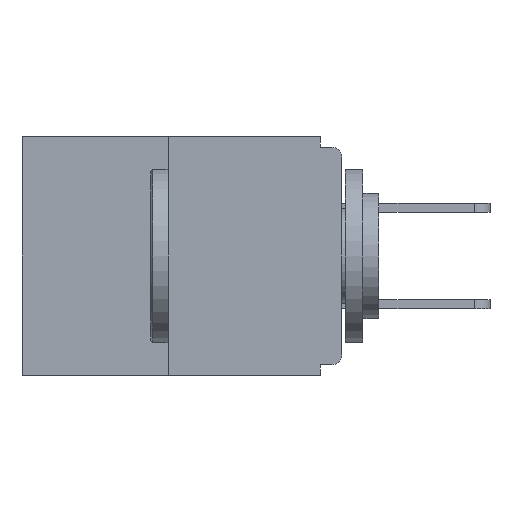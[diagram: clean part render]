
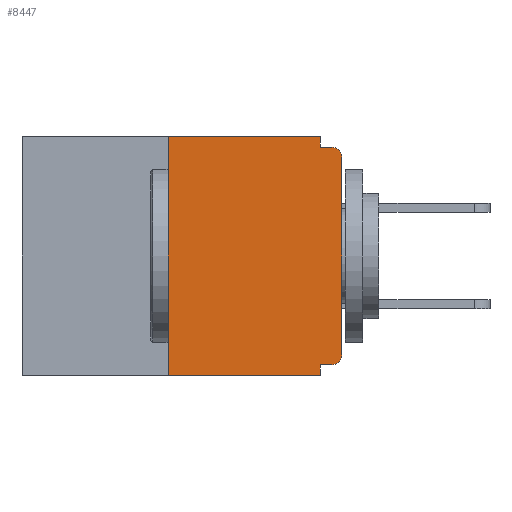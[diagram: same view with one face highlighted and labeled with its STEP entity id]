
A CAD part, left-side view. The second image highlights one B-rep face of the part: STEP entity #8447.
In plain terms, the highlighted planar face has unit normal (-1, 0, 0).
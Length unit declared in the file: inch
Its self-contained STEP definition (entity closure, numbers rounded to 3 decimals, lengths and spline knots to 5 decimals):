
#689 = LINE ( 'NONE', #3879, #4728 ) ;
#1601 = DIRECTION ( 'NONE',  ( 0., 0., -1. ) ) ;
#1775 = VECTOR ( 'NONE', #1817, 39.37008 ) ;
#1817 = DIRECTION ( 'NONE',  ( 0., 0., 1. ) ) ;
#2241 = LINE ( 'NONE', #26391, #17883 ) ;
#3178 = VECTOR ( 'NONE', #17143, 39.37008 ) ;
#3440 = CARTESIAN_POINT ( 'NONE',  ( 0., 0.25, 0. ) ) ;
#3879 = CARTESIAN_POINT ( 'NONE',  ( 0., 0.46, -0.343 ) ) ;
#4091 = LINE ( 'NONE', #7832, #24764 ) ;
#4187 = ORIENTED_EDGE ( 'NONE', *, *, #27512, .F. ) ;
#4209 = DIRECTION ( 'NONE',  ( 0., -1., 0. ) ) ;
#4233 = ORIENTED_EDGE ( 'NONE', *, *, #19570, .F. ) ;
#4329 = CIRCLE ( 'NONE', #6587, 0.015 ) ;
#4728 = VECTOR ( 'NONE', #22437, 39.37008 ) ;
#4934 = EDGE_CURVE ( 'NONE', #9540, #29131, #4329, .T. ) ;
#5716 = CIRCLE ( 'NONE', #19223, 0.015 ) ;
#5786 = EDGE_LOOP ( 'NONE', ( #4187, #16354, #23228, #4233, #12359, #24654, #11772, #14739, #16747, #27413 ) ) ;
#5897 = VERTEX_POINT ( 'NONE', #22244 ) ;
#6348 = CARTESIAN_POINT ( 'NONE',  ( 0., 0., -0.015 ) ) ;
#6507 = DIRECTION ( 'NONE',  ( -1., 0., 0. ) ) ;
#6508 = CARTESIAN_POINT ( 'NONE',  ( 0., 0.031, 0. ) ) ;
#6549 = CARTESIAN_POINT ( 'NONE',  ( 0., 0.015, -0.328 ) ) ;
#6587 = AXIS2_PLACEMENT_3D ( 'NONE', #12841, #15266, #22357 ) ;
#6956 = VERTEX_POINT ( 'NONE', #29626 ) ;
#7216 = VERTEX_POINT ( 'NONE', #6508 ) ;
#7235 = VECTOR ( 'NONE', #4209, 39.37008 ) ;
#7832 = CARTESIAN_POINT ( 'NONE',  ( 0., 0.25, 0. ) ) ;
#7849 = CARTESIAN_POINT ( 'NONE',  ( 0., 0.031, -0.343 ) ) ;
#8447 = ADVANCED_FACE ( 'NONE', ( #19370 ), #21222, .F. ) ;
#9181 = VECTOR ( 'NONE', #25847, 39.37008 ) ;
#9540 = VERTEX_POINT ( 'NONE', #6549 ) ;
#9655 = EDGE_CURVE ( 'NONE', #9540, #15484, #25860, .T. ) ;
#10981 = VERTEX_POINT ( 'NONE', #7849 ) ;
#11085 = EDGE_CURVE ( 'NONE', #28383, #5897, #5716, .T. ) ;
#11482 = EDGE_CURVE ( 'NONE', #7216, #26706, #20924, .T. ) ;
#11772 = ORIENTED_EDGE ( 'NONE', *, *, #20903, .T. ) ;
#11995 = DIRECTION ( 'NONE',  ( 1., 0., 0. ) ) ;
#12359 = ORIENTED_EDGE ( 'NONE', *, *, #9655, .F. ) ;
#12841 = CARTESIAN_POINT ( 'NONE',  ( 0., 0.015, -0.313 ) ) ;
#13002 = CARTESIAN_POINT ( 'NONE',  ( 0., 0.015, -0.03 ) ) ;
#13765 = CARTESIAN_POINT ( 'NONE',  ( 0., 0.031, -0.328 ) ) ;
#13858 = VERTEX_POINT ( 'NONE', #3440 ) ;
#14214 = CARTESIAN_POINT ( 'NONE',  ( 0., 0., -0.328 ) ) ;
#14515 = CARTESIAN_POINT ( 'NONE',  ( 0., 0.46, 0. ) ) ;
#14739 = ORIENTED_EDGE ( 'NONE', *, *, #11085, .T. ) ;
#14785 = CARTESIAN_POINT ( 'NONE',  ( 0., 0.46, 0. ) ) ;
#15065 = DIRECTION ( 'NONE',  ( 0., 0., -1. ) ) ;
#15266 = DIRECTION ( 'NONE',  ( -1., 0., 0. ) ) ;
#15484 = VERTEX_POINT ( 'NONE', #13765 ) ;
#15925 = DIRECTION ( 'NONE',  ( 0., 0., -1. ) ) ;
#16354 = ORIENTED_EDGE ( 'NONE', *, *, #19611, .F. ) ;
#16747 = ORIENTED_EDGE ( 'NONE', *, *, #18200, .F. ) ;
#16863 = DIRECTION ( 'NONE',  ( 0., 0., -1. ) ) ;
#17143 = DIRECTION ( 'NONE',  ( 0., -1., 0. ) ) ;
#17883 = VECTOR ( 'NONE', #15065, 39.37008 ) ;
#17981 = CARTESIAN_POINT ( 'NONE',  ( 0., 0., 0. ) ) ;
#18200 = EDGE_CURVE ( 'NONE', #26706, #5897, #27520, .T. ) ;
#18285 = CARTESIAN_POINT ( 'NONE',  ( 0., 0., -0.313 ) ) ;
#19223 = AXIS2_PLACEMENT_3D ( 'NONE', #13002, #6507, #15925 ) ;
#19370 = FACE_OUTER_BOUND ( 'NONE', #5786, .T. ) ;
#19570 = EDGE_CURVE ( 'NONE', #15484, #10981, #2241, .T. ) ;
#19611 = EDGE_CURVE ( 'NONE', #6956, #13858, #4091, .T. ) ;
#20903 = EDGE_CURVE ( 'NONE', #29131, #28383, #27178, .T. ) ;
#20924 = LINE ( 'NONE', #24845, #21649 ) ;
#20941 = EDGE_CURVE ( 'NONE', #6956, #10981, #689, .T. ) ;
#21222 = PLANE ( 'NONE',  #27089 ) ;
#21455 = CARTESIAN_POINT ( 'NONE',  ( 0., 0., -0.03 ) ) ;
#21649 = VECTOR ( 'NONE', #1601, 39.37008 ) ;
#22244 = CARTESIAN_POINT ( 'NONE',  ( 0., 0.015, -0.015 ) ) ;
#22357 = DIRECTION ( 'NONE',  ( 0., 0., -1. ) ) ;
#22437 = DIRECTION ( 'NONE',  ( 0., -1., 0. ) ) ;
#23228 = ORIENTED_EDGE ( 'NONE', *, *, #20941, .T. ) ;
#24654 = ORIENTED_EDGE ( 'NONE', *, *, #4934, .T. ) ;
#24764 = VECTOR ( 'NONE', #28693, 39.37008 ) ;
#24845 = CARTESIAN_POINT ( 'NONE',  ( 0., 0.031, 0. ) ) ;
#25847 = DIRECTION ( 'NONE',  ( 0., 1., 0. ) ) ;
#25860 = LINE ( 'NONE', #14214, #9181 ) ;
#26326 = CARTESIAN_POINT ( 'NONE',  ( 0., 0.031, -0.015 ) ) ;
#26391 = CARTESIAN_POINT ( 'NONE',  ( 0., 0.031, -0.343 ) ) ;
#26706 = VERTEX_POINT ( 'NONE', #26326 ) ;
#27089 = AXIS2_PLACEMENT_3D ( 'NONE', #14515, #11995, #16863 ) ;
#27178 = LINE ( 'NONE', #17981, #1775 ) ;
#27413 = ORIENTED_EDGE ( 'NONE', *, *, #11482, .F. ) ;
#27493 = LINE ( 'NONE', #14785, #3178 ) ;
#27512 = EDGE_CURVE ( 'NONE', #13858, #7216, #27493, .T. ) ;
#27520 = LINE ( 'NONE', #6348, #7235 ) ;
#28383 = VERTEX_POINT ( 'NONE', #21455 ) ;
#28693 = DIRECTION ( 'NONE',  ( 0., 0., 1. ) ) ;
#29131 = VERTEX_POINT ( 'NONE', #18285 ) ;
#29626 = CARTESIAN_POINT ( 'NONE',  ( 0., 0.25, -0.343 ) ) ;
